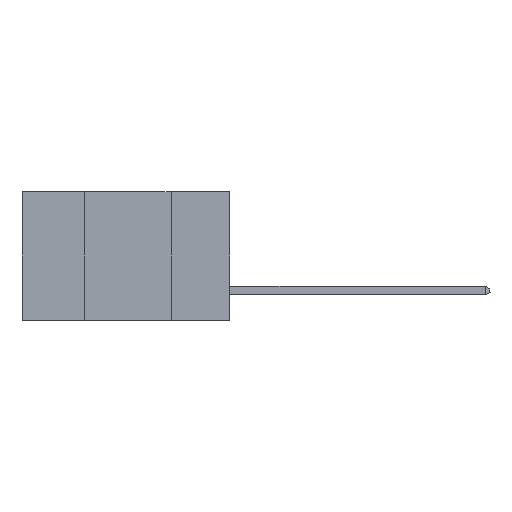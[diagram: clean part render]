
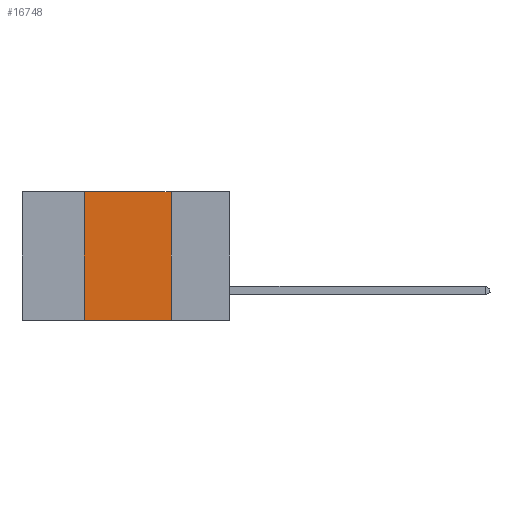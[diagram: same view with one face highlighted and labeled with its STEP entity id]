
A CAD part, left-side view. The second image highlights one B-rep face of the part: STEP entity #16748.
In plain terms, the highlighted planar face has unit normal (-1, 0, 0).
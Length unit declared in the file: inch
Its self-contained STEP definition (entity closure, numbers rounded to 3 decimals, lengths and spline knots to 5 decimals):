
#1891 = EDGE_CURVE ( 'NONE', #16622, #2082, #9372, .T. ) ;
#2082 = VERTEX_POINT ( 'NONE', #2215 ) ;
#2117 = DIRECTION ( 'NONE',  ( 0., -1., 0. ) ) ;
#2215 = CARTESIAN_POINT ( 'NONE',  ( 0., 0.17, -0.37 ) ) ;
#3832 = VERTEX_POINT ( 'NONE', #17623 ) ;
#3936 = DIRECTION ( 'NONE',  ( 0., -1., 0. ) ) ;
#4508 = EDGE_CURVE ( 'NONE', #16622, #3832, #6972, .T. ) ;
#4633 = FACE_OUTER_BOUND ( 'NONE', #12480, .T. ) ;
#5152 = CARTESIAN_POINT ( 'NONE',  ( 0., 0.42, -0.37 ) ) ;
#5518 = DIRECTION ( 'NONE',  ( 1., 0., 0. ) ) ;
#5779 = ORIENTED_EDGE ( 'NONE', *, *, #9462, .F. ) ;
#5874 = CARTESIAN_POINT ( 'NONE',  ( 0., 0.17, 0. ) ) ;
#6119 = VECTOR ( 'NONE', #2117, 39.37008 ) ;
#6846 = DIRECTION ( 'NONE',  ( 0., 0., 1. ) ) ;
#6870 = CARTESIAN_POINT ( 'NONE',  ( 0., 0.6, -0.37 ) ) ;
#6972 = LINE ( 'NONE', #9648, #13837 ) ;
#7585 = LINE ( 'NONE', #8728, #6119 ) ;
#8135 = DIRECTION ( 'NONE',  ( 0., 0., -1. ) ) ;
#8728 = CARTESIAN_POINT ( 'NONE',  ( 0., 0.6, 0. ) ) ;
#9267 = AXIS2_PLACEMENT_3D ( 'NONE', #16567, #5518, #8135 ) ;
#9372 = LINE ( 'NONE', #6870, #11547 ) ;
#9462 = EDGE_CURVE ( 'NONE', #10476, #2082, #10475, .T. ) ;
#9648 = CARTESIAN_POINT ( 'NONE',  ( 0., 0.42, 0. ) ) ;
#10475 = LINE ( 'NONE', #5874, #11146 ) ;
#10476 = VERTEX_POINT ( 'NONE', #11907 ) ;
#11044 = PLANE ( 'NONE',  #9267 ) ;
#11146 = VECTOR ( 'NONE', #15334, 39.37008 ) ;
#11547 = VECTOR ( 'NONE', #3936, 39.37008 ) ;
#11907 = CARTESIAN_POINT ( 'NONE',  ( 0., 0.17, 0. ) ) ;
#12480 = EDGE_LOOP ( 'NONE', ( #5779, #12713, #17216, #13858 ) ) ;
#12713 = ORIENTED_EDGE ( 'NONE', *, *, #12938, .F. ) ;
#12938 = EDGE_CURVE ( 'NONE', #3832, #10476, #7585, .T. ) ;
#13837 = VECTOR ( 'NONE', #6846, 39.37008 ) ;
#13858 = ORIENTED_EDGE ( 'NONE', *, *, #1891, .T. ) ;
#15334 = DIRECTION ( 'NONE',  ( 0., 0., -1. ) ) ;
#16567 = CARTESIAN_POINT ( 'NONE',  ( 0., 0.6, 0. ) ) ;
#16622 = VERTEX_POINT ( 'NONE', #5152 ) ;
#16748 = ADVANCED_FACE ( 'NONE', ( #4633 ), #11044, .F. ) ;
#17216 = ORIENTED_EDGE ( 'NONE', *, *, #4508, .F. ) ;
#17623 = CARTESIAN_POINT ( 'NONE',  ( 0., 0.42, 0. ) ) ;
